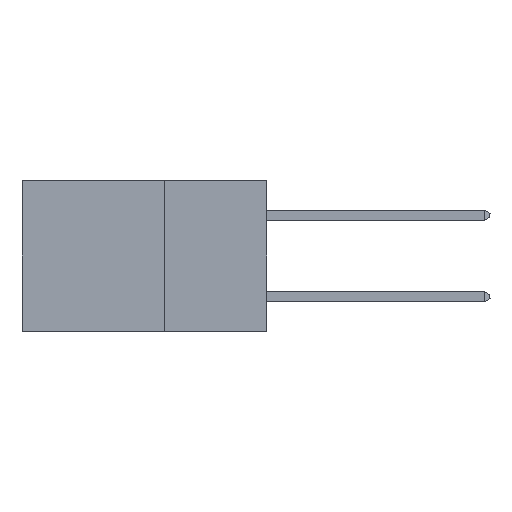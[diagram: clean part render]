
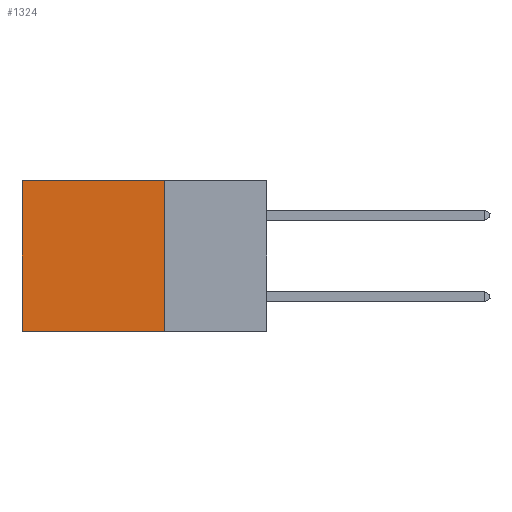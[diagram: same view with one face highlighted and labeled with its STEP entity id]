
A CAD part, left-side view. The second image highlights one B-rep face of the part: STEP entity #1324.
In plain terms, the highlighted planar face has unit normal (-1, 0, 0).
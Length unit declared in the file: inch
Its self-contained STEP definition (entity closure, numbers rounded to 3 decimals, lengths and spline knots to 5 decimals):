
#587 = VERTEX_POINT ( 'NONE', #37930 ) ;
#1291 = LINE ( 'NONE', #4333, #37943 ) ;
#1324 = ADVANCED_FACE ( 'NONE', ( #45594 ), #45246, .F. ) ;
#2151 = CARTESIAN_POINT ( 'NONE',  ( 0.2875, 0.25, 0. ) ) ;
#2681 = DIRECTION ( 'NONE',  ( 0., 0., -1. ) ) ;
#2985 = ORIENTED_EDGE ( 'NONE', *, *, #20806, .T. ) ;
#4333 = CARTESIAN_POINT ( 'NONE',  ( 0.2875, 0.25, 0. ) ) ;
#4374 = EDGE_CURVE ( 'NONE', #20597, #22302, #44245, .T. ) ;
#6278 = DIRECTION ( 'NONE',  ( 0., 0., -1. ) ) ;
#6483 = VECTOR ( 'NONE', #23374, 39.37008 ) ;
#9068 = AXIS2_PLACEMENT_3D ( 'NONE', #23913, #27530, #6278 ) ;
#10440 = VERTEX_POINT ( 'NONE', #28454 ) ;
#11321 = DIRECTION ( 'NONE',  ( 0., 1., 0. ) ) ;
#14487 = CARTESIAN_POINT ( 'NONE',  ( 0.2875, 0.25, -0.37 ) ) ;
#17380 = ORIENTED_EDGE ( 'NONE', *, *, #4374, .F. ) ;
#19287 = CARTESIAN_POINT ( 'NONE',  ( 0.2875, 0.25, 0. ) ) ;
#20597 = VERTEX_POINT ( 'NONE', #19287 ) ;
#20806 = EDGE_CURVE ( 'NONE', #10440, #587, #29478, .T. ) ;
#22302 = VERTEX_POINT ( 'NONE', #14487 ) ;
#23223 = EDGE_CURVE ( 'NONE', #22302, #587, #43113, .T. ) ;
#23374 = DIRECTION ( 'NONE',  ( 0., 0., -1. ) ) ;
#23913 = CARTESIAN_POINT ( 'NONE',  ( 0.2875, 0.25, 0. ) ) ;
#24178 = VECTOR ( 'NONE', #26231, 39.37008 ) ;
#25642 = EDGE_CURVE ( 'NONE', #20597, #10440, #1291, .T. ) ;
#26231 = DIRECTION ( 'NONE',  ( 0., 1., 0. ) ) ;
#27236 = VECTOR ( 'NONE', #2681, 39.37008 ) ;
#27530 = DIRECTION ( 'NONE',  ( 1., 0., 0. ) ) ;
#27957 = ORIENTED_EDGE ( 'NONE', *, *, #23223, .F. ) ;
#28454 = CARTESIAN_POINT ( 'NONE',  ( 0.2875, 0.6, 0. ) ) ;
#29478 = LINE ( 'NONE', #30925, #27236 ) ;
#30925 = CARTESIAN_POINT ( 'NONE',  ( 0.2875, 0.6, 0. ) ) ;
#36989 = CARTESIAN_POINT ( 'NONE',  ( 0.2875, 0.25, -0.37 ) ) ;
#37019 = EDGE_LOOP ( 'NONE', ( #2985, #27957, #17380, #40340 ) ) ;
#37930 = CARTESIAN_POINT ( 'NONE',  ( 0.2875, 0.6, -0.37 ) ) ;
#37943 = VECTOR ( 'NONE', #11321, 39.37008 ) ;
#40340 = ORIENTED_EDGE ( 'NONE', *, *, #25642, .T. ) ;
#43113 = LINE ( 'NONE', #36989, #24178 ) ;
#44245 = LINE ( 'NONE', #2151, #6483 ) ;
#45246 = PLANE ( 'NONE',  #9068 ) ;
#45594 = FACE_OUTER_BOUND ( 'NONE', #37019, .T. ) ;
